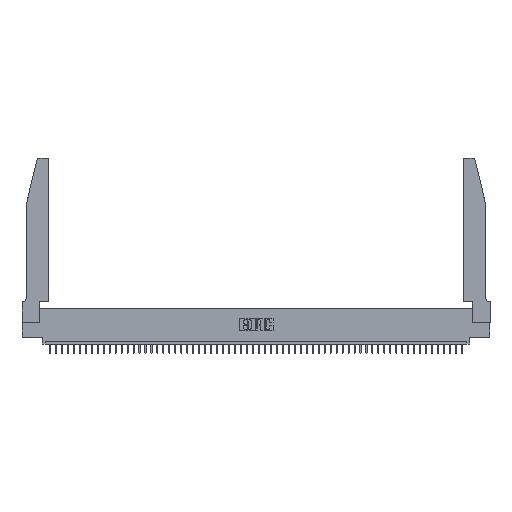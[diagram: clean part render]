
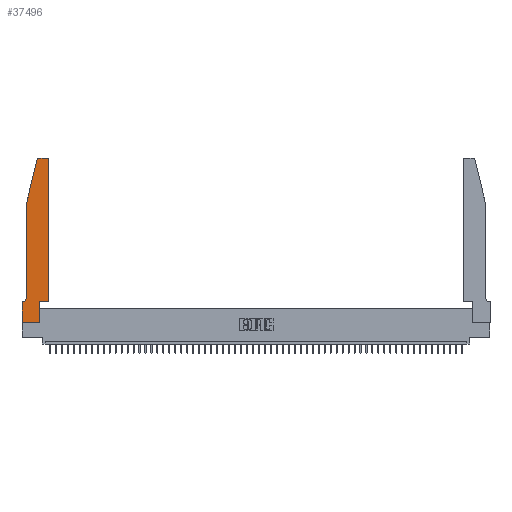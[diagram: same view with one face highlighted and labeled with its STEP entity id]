
A CAD part, top view. The second image highlights one B-rep face of the part: STEP entity #37496.
In plain terms, the highlighted planar face has unit normal (0, 0, 1).
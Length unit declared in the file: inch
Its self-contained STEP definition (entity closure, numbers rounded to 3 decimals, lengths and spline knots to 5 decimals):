
#300 = ORIENTED_EDGE ( 'NONE', *, *, #15050, .T. ) ;
#631 = VECTOR ( 'NONE', #33797, 39.37008 ) ;
#908 = EDGE_CURVE ( 'NONE', #5772, #11225, #48820, .T. ) ;
#988 = CARTESIAN_POINT ( 'NONE',  ( 0.2865, 0., 0.37 ) ) ;
#1598 = CARTESIAN_POINT ( 'NONE',  ( 0.0755, 0.42, 0.37 ) ) ;
#2779 = VECTOR ( 'NONE', #42066, 39.37008 ) ;
#2926 = DIRECTION ( 'NONE',  ( 1., 0., 0. ) ) ;
#3916 = DIRECTION ( 'NONE',  ( 0., 0., 1. ) ) ;
#4192 = CARTESIAN_POINT ( 'NONE',  ( 0.4205, 2.75, 0.37 ) ) ;
#4769 = LINE ( 'NONE', #35605, #24260 ) ;
#5257 = LINE ( 'NONE', #48591, #9130 ) ;
#5466 = VECTOR ( 'NONE', #9512, 39.37008 ) ;
#5568 = AXIS2_PLACEMENT_3D ( 'NONE', #52719, #27737, #2926 ) ;
#5682 = CARTESIAN_POINT ( 'NONE',  ( 0., 0., 0.37 ) ) ;
#5772 = VERTEX_POINT ( 'NONE', #36307 ) ;
#6075 = CARTESIAN_POINT ( 'NONE',  ( 0.4505, 0.35, 0.37 ) ) ;
#6374 = ORIENTED_EDGE ( 'NONE', *, *, #40564, .T. ) ;
#6931 = DIRECTION ( 'NONE',  ( 1., 0., 0. ) ) ;
#7004 = CARTESIAN_POINT ( 'NONE',  ( 0.4505, 2.72, 0.37 ) ) ;
#7397 = EDGE_CURVE ( 'NONE', #40815, #8781, #35378, .T. ) ;
#7893 = AXIS2_PLACEMENT_3D ( 'NONE', #16558, #3916, #29438 ) ;
#8781 = VERTEX_POINT ( 'NONE', #5682 ) ;
#8941 = CARTESIAN_POINT ( 'NONE',  ( 0.0055, 0.42, 0.37 ) ) ;
#9018 = ORIENTED_EDGE ( 'NONE', *, *, #39805, .T. ) ;
#9130 = VECTOR ( 'NONE', #6931, 39.37008 ) ;
#9512 = DIRECTION ( 'NONE',  ( 1., 0., 0. ) ) ;
#9981 = AXIS2_PLACEMENT_3D ( 'NONE', #8941, #50784, #21475 ) ;
#10935 = CARTESIAN_POINT ( 'NONE',  ( 0.0755, 2., 0.37 ) ) ;
#11225 = VERTEX_POINT ( 'NONE', #10935 ) ;
#12648 = ORIENTED_EDGE ( 'NONE', *, *, #13423, .T. ) ;
#13256 = EDGE_CURVE ( 'NONE', #50362, #51842, #29511, .T. ) ;
#13423 = EDGE_CURVE ( 'NONE', #8781, #27805, #43200, .T. ) ;
#13489 = CARTESIAN_POINT ( 'NONE',  ( 0., 0., 0.37 ) ) ;
#14253 = CIRCLE ( 'NONE', #17078, 0.03 ) ;
#15050 = EDGE_CURVE ( 'NONE', #52374, #50362, #5257, .T. ) ;
#15445 = VERTEX_POINT ( 'NONE', #49944 ) ;
#15656 = EDGE_CURVE ( 'NONE', #19591, #15445, #52018, .T. ) ;
#15893 = VECTOR ( 'NONE', #35710, 39.37008 ) ;
#16558 = CARTESIAN_POINT ( 'NONE',  ( 0., 0.35, 0.37 ) ) ;
#16875 = CARTESIAN_POINT ( 'NONE',  ( 0.0755, 2., 0.37 ) ) ;
#17078 = AXIS2_PLACEMENT_3D ( 'NONE', #31087, #35504, #22737 ) ;
#17957 = ORIENTED_EDGE ( 'NONE', *, *, #15656, .T. ) ;
#18089 = CARTESIAN_POINT ( 'NONE',  ( 0.0755, 2., 0.37 ) ) ;
#18936 = DIRECTION ( 'NONE',  ( 0., -1., 0. ) ) ;
#19425 = ORIENTED_EDGE ( 'NONE', *, *, #53414, .T. ) ;
#19591 = VERTEX_POINT ( 'NONE', #1598 ) ;
#20176 = CARTESIAN_POINT ( 'NONE',  ( 0.2865, 0.35, 0.37 ) ) ;
#20800 = EDGE_CURVE ( 'NONE', #27805, #52374, #30275, .T. ) ;
#21475 = DIRECTION ( 'NONE',  ( -1., 0., 0. ) ) ;
#22737 = DIRECTION ( 'NONE',  ( 1., 0., 0. ) ) ;
#23325 = VECTOR ( 'NONE', #25928, 39.37008 ) ;
#24260 = VECTOR ( 'NONE', #36516, 39.37008 ) ;
#25928 = DIRECTION ( 'NONE',  ( 0., -1., 0. ) ) ;
#26447 = FACE_OUTER_BOUND ( 'NONE', #36798, .T. ) ;
#27083 = CARTESIAN_POINT ( 'NONE',  ( 0., 0., 0.37 ) ) ;
#27737 = DIRECTION ( 'NONE',  ( 0., 0., 1. ) ) ;
#27805 = VERTEX_POINT ( 'NONE', #988 ) ;
#28381 = VERTEX_POINT ( 'NONE', #39947 ) ;
#29135 = LINE ( 'NONE', #16875, #23325 ) ;
#29265 = PLANE ( 'NONE',  #7893 ) ;
#29438 = DIRECTION ( 'NONE',  ( 1., 0., 0. ) ) ;
#29511 = LINE ( 'NONE', #6075, #15893 ) ;
#29920 = CARTESIAN_POINT ( 'NONE',  ( 0., 0.35, 0.37 ) ) ;
#30275 = LINE ( 'NONE', #39386, #51169 ) ;
#31087 = CARTESIAN_POINT ( 'NONE',  ( 0.4205, 2.72, 0.37 ) ) ;
#32960 = ORIENTED_EDGE ( 'NONE', *, *, #34903, .T. ) ;
#33797 = DIRECTION ( 'NONE',  ( -0.239, -0.971, 0. ) ) ;
#34903 = EDGE_CURVE ( 'NONE', #11225, #19591, #29135, .T. ) ;
#35378 = LINE ( 'NONE', #27083, #49772 ) ;
#35504 = DIRECTION ( 'NONE',  ( 0., 0., 1. ) ) ;
#35605 = CARTESIAN_POINT ( 'NONE',  ( 0.0755, 0.35, 0.37 ) ) ;
#35710 = DIRECTION ( 'NONE',  ( 0., 1., 0. ) ) ;
#36307 = CARTESIAN_POINT ( 'NONE',  ( 0.25487, 2.72718, 0.37 ) ) ;
#36516 = DIRECTION ( 'NONE',  ( -1., 0., 0. ) ) ;
#36798 = EDGE_LOOP ( 'NONE', ( #52707, #6374, #37959, #32960, #17957, #9018, #50260, #12648, #43109, #300, #53300, #19425 ) ) ;
#37496 = ADVANCED_FACE ( 'NONE', ( #26447 ), #29265, .T. ) ;
#37579 = VERTEX_POINT ( 'NONE', #4192 ) ;
#37959 = ORIENTED_EDGE ( 'NONE', *, *, #908, .T. ) ;
#38830 = DIRECTION ( 'NONE',  ( 0., 1., 0. ) ) ;
#39386 = CARTESIAN_POINT ( 'NONE',  ( 0.2865, 0.35, 0.37 ) ) ;
#39805 = EDGE_CURVE ( 'NONE', #15445, #40815, #4769, .T. ) ;
#39947 = CARTESIAN_POINT ( 'NONE',  ( 0.284, 2.75, 0.37 ) ) ;
#40564 = EDGE_CURVE ( 'NONE', #28381, #5772, #51515, .T. ) ;
#40815 = VERTEX_POINT ( 'NONE', #29920 ) ;
#41169 = LINE ( 'NONE', #50103, #2779 ) ;
#42066 = DIRECTION ( 'NONE',  ( -1., 0., 0. ) ) ;
#43109 = ORIENTED_EDGE ( 'NONE', *, *, #20800, .T. ) ;
#43200 = LINE ( 'NONE', #13489, #5466 ) ;
#48591 = CARTESIAN_POINT ( 'NONE',  ( 0.4505, 0.35, 0.37 ) ) ;
#48820 = LINE ( 'NONE', #18089, #631 ) ;
#49772 = VECTOR ( 'NONE', #18936, 39.37008 ) ;
#49944 = CARTESIAN_POINT ( 'NONE',  ( 0.0055, 0.35, 0.37 ) ) ;
#50103 = CARTESIAN_POINT ( 'NONE',  ( 0.2605, 2.75, 0.37 ) ) ;
#50260 = ORIENTED_EDGE ( 'NONE', *, *, #7397, .T. ) ;
#50362 = VERTEX_POINT ( 'NONE', #51131 ) ;
#50784 = DIRECTION ( 'NONE',  ( 0., 0., -1. ) ) ;
#51131 = CARTESIAN_POINT ( 'NONE',  ( 0.4505, 0.35, 0.37 ) ) ;
#51169 = VECTOR ( 'NONE', #38830, 39.37008 ) ;
#51515 = CIRCLE ( 'NONE', #5568, 0.03 ) ;
#51842 = VERTEX_POINT ( 'NONE', #7004 ) ;
#51971 = EDGE_CURVE ( 'NONE', #37579, #28381, #41169, .T. ) ;
#52018 = CIRCLE ( 'NONE', #9981, 0.07 ) ;
#52374 = VERTEX_POINT ( 'NONE', #20176 ) ;
#52707 = ORIENTED_EDGE ( 'NONE', *, *, #51971, .T. ) ;
#52719 = CARTESIAN_POINT ( 'NONE',  ( 0.284, 2.72, 0.37 ) ) ;
#53300 = ORIENTED_EDGE ( 'NONE', *, *, #13256, .T. ) ;
#53414 = EDGE_CURVE ( 'NONE', #51842, #37579, #14253, .T. ) ;
